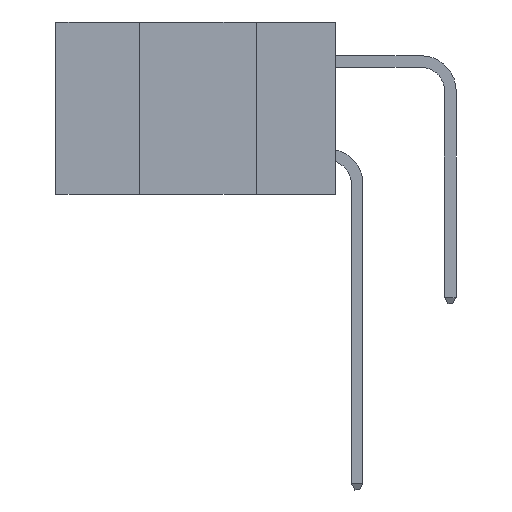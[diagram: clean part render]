
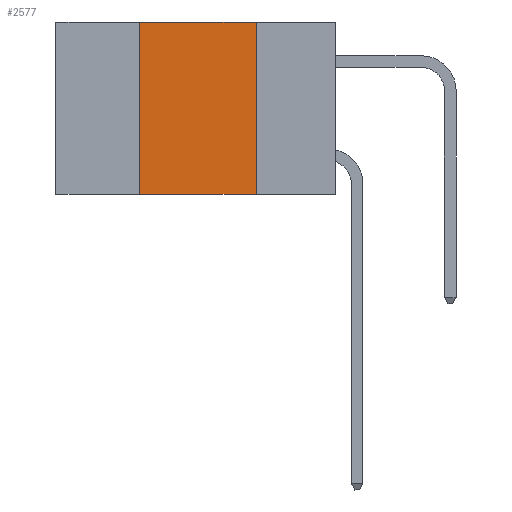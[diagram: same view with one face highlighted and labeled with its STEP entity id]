
A CAD part, left-side view. The second image highlights one B-rep face of the part: STEP entity #2577.
In plain terms, the highlighted planar face has unit normal (-1, 0, 0).
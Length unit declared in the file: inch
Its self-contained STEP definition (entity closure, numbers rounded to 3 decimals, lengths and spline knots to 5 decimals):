
#628 = EDGE_CURVE ( 'NONE', #3803, #8779, #2358, .T. ) ;
#936 = VECTOR ( 'NONE', #9390, 39.37008 ) ;
#1006 = ORIENTED_EDGE ( 'NONE', *, *, #628, .F. ) ;
#1532 = CARTESIAN_POINT ( 'NONE',  ( 0., 0.42, 0. ) ) ;
#1599 = ORIENTED_EDGE ( 'NONE', *, *, #11880, .F. ) ;
#2342 = LINE ( 'NONE', #7809, #936 ) ;
#2358 = LINE ( 'NONE', #2518, #13325 ) ;
#2518 = CARTESIAN_POINT ( 'NONE',  ( 0., 0.17, 0. ) ) ;
#2577 = ADVANCED_FACE ( 'NONE', ( #10187 ), #7333, .F. ) ;
#2707 = CARTESIAN_POINT ( 'NONE',  ( 0., 0.6, -0.37 ) ) ;
#2864 = LINE ( 'NONE', #1532, #6223 ) ;
#2916 = AXIS2_PLACEMENT_3D ( 'NONE', #11335, #5988, #13020 ) ;
#3803 = VERTEX_POINT ( 'NONE', #7332 ) ;
#4735 = EDGE_CURVE ( 'NONE', #11277, #3803, #2342, .T. ) ;
#4991 = ORIENTED_EDGE ( 'NONE', *, *, #13276, .T. ) ;
#5988 = DIRECTION ( 'NONE',  ( 1., 0., 0. ) ) ;
#6223 = VECTOR ( 'NONE', #9664, 39.37008 ) ;
#7015 = CARTESIAN_POINT ( 'NONE',  ( 0., 0.42, 0. ) ) ;
#7332 = CARTESIAN_POINT ( 'NONE',  ( 0., 0.17, 0. ) ) ;
#7333 = PLANE ( 'NONE',  #2916 ) ;
#7809 = CARTESIAN_POINT ( 'NONE',  ( 0., 0.6, 0. ) ) ;
#8080 = DIRECTION ( 'NONE',  ( 0., 0., -1. ) ) ;
#8253 = EDGE_LOOP ( 'NONE', ( #1006, #12204, #1599, #4991 ) ) ;
#8779 = VERTEX_POINT ( 'NONE', #12674 ) ;
#8818 = CARTESIAN_POINT ( 'NONE',  ( 0., 0.42, -0.37 ) ) ;
#9390 = DIRECTION ( 'NONE',  ( 0., -1., 0. ) ) ;
#9664 = DIRECTION ( 'NONE',  ( 0., 0., 1. ) ) ;
#10187 = FACE_OUTER_BOUND ( 'NONE', #8253, .T. ) ;
#11277 = VERTEX_POINT ( 'NONE', #7015 ) ;
#11335 = CARTESIAN_POINT ( 'NONE',  ( 0., 0.6, 0. ) ) ;
#11880 = EDGE_CURVE ( 'NONE', #16553, #11277, #2864, .T. ) ;
#12163 = LINE ( 'NONE', #2707, #13042 ) ;
#12204 = ORIENTED_EDGE ( 'NONE', *, *, #4735, .F. ) ;
#12674 = CARTESIAN_POINT ( 'NONE',  ( 0., 0.17, -0.37 ) ) ;
#13020 = DIRECTION ( 'NONE',  ( 0., 0., -1. ) ) ;
#13042 = VECTOR ( 'NONE', #13678, 39.37008 ) ;
#13276 = EDGE_CURVE ( 'NONE', #16553, #8779, #12163, .T. ) ;
#13325 = VECTOR ( 'NONE', #8080, 39.37008 ) ;
#13678 = DIRECTION ( 'NONE',  ( 0., -1., 0. ) ) ;
#16553 = VERTEX_POINT ( 'NONE', #8818 ) ;
